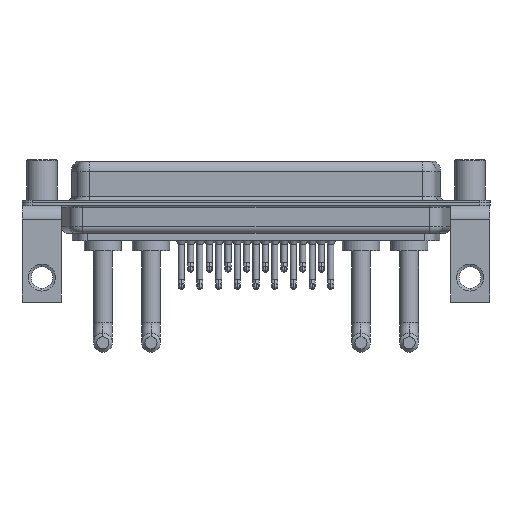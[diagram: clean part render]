
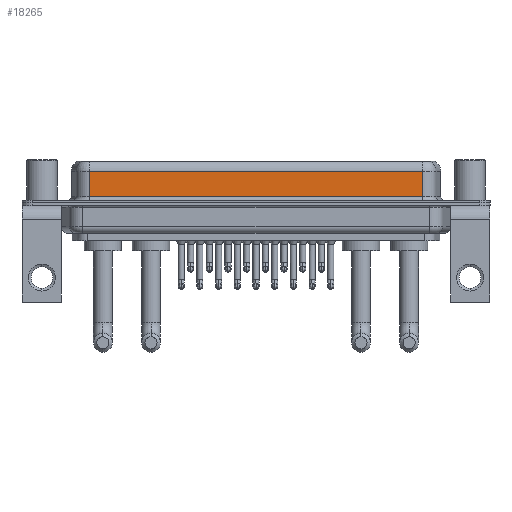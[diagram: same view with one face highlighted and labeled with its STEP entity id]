
A CAD part, front view. The second image highlights one B-rep face of the part: STEP entity #18265.
In plain terms, the highlighted planar face has unit normal (0, -1, 0).
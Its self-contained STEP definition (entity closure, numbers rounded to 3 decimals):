
#540 = VECTOR ( 'NONE', #15277, 1000. ) ;
#2119 = EDGE_LOOP ( 'NONE', ( #23455, #6418, #21085, #22426 ) ) ;
#3664 = AXIS2_PLACEMENT_3D ( 'NONE', #14513, #5076, #12653 ) ;
#4736 = DIRECTION ( 'NONE',  ( -1., 0., 0. ) ) ;
#5076 = DIRECTION ( 'NONE',  ( 0., 1., 0. ) ) ;
#5312 = CARTESIAN_POINT ( 'NONE',  ( 56.462, -3.95, 0.9 ) ) ;
#5611 = CARTESIAN_POINT ( 'NONE',  ( 56.462, -3.95, 6.4 ) ) ;
#6130 = LINE ( 'NONE', #19630, #22427 ) ;
#6417 = EDGE_CURVE ( 'NONE', #24205, #14981, #13853, .T. ) ;
#6418 = ORIENTED_EDGE ( 'NONE', *, *, #17570, .T. ) ;
#7288 = VERTEX_POINT ( 'NONE', #24466 ) ;
#8151 = CARTESIAN_POINT ( 'NONE',  ( 7.038, -3.95, 6.4 ) ) ;
#8830 = PLANE ( 'NONE',  #3664 ) ;
#9139 = CARTESIAN_POINT ( 'NONE',  ( 56.462, -3.95, 4.65 ) ) ;
#9355 = LINE ( 'NONE', #5611, #540 ) ;
#10412 = CARTESIAN_POINT ( 'NONE',  ( 7.038, -3.95, 0.9 ) ) ;
#10696 = FACE_OUTER_BOUND ( 'NONE', #2119, .T. ) ;
#11996 = DIRECTION ( 'NONE',  ( 1., 0., 0. ) ) ;
#12653 = DIRECTION ( 'NONE',  ( 0., 0., 1. ) ) ;
#13569 = EDGE_CURVE ( 'NONE', #17259, #14981, #9355, .T. ) ;
#13853 = LINE ( 'NONE', #23278, #16533 ) ;
#14073 = LINE ( 'NONE', #8151, #21169 ) ;
#14354 = EDGE_CURVE ( 'NONE', #7288, #24205, #14073, .T. ) ;
#14513 = CARTESIAN_POINT ( 'NONE',  ( 56.462, -3.95, 6.4 ) ) ;
#14981 = VERTEX_POINT ( 'NONE', #5312 ) ;
#15277 = DIRECTION ( 'NONE',  ( 0., 0., -1. ) ) ;
#16533 = VECTOR ( 'NONE', #11996, 1000. ) ;
#17259 = VERTEX_POINT ( 'NONE', #9139 ) ;
#17570 = EDGE_CURVE ( 'NONE', #17259, #7288, #6130, .T. ) ;
#18265 = ADVANCED_FACE ( 'NONE', ( #10696 ), #8830, .F. ) ;
#19630 = CARTESIAN_POINT ( 'NONE',  ( 56.462, -3.95, 4.65 ) ) ;
#21085 = ORIENTED_EDGE ( 'NONE', *, *, #14354, .T. ) ;
#21169 = VECTOR ( 'NONE', #21394, 1000. ) ;
#21394 = DIRECTION ( 'NONE',  ( 0., 0., -1. ) ) ;
#22426 = ORIENTED_EDGE ( 'NONE', *, *, #6417, .T. ) ;
#22427 = VECTOR ( 'NONE', #4736, 1000. ) ;
#23278 = CARTESIAN_POINT ( 'NONE',  ( 56.462, -3.95, 0.9 ) ) ;
#23455 = ORIENTED_EDGE ( 'NONE', *, *, #13569, .F. ) ;
#24205 = VERTEX_POINT ( 'NONE', #10412 ) ;
#24466 = CARTESIAN_POINT ( 'NONE',  ( 7.038, -3.95, 4.65 ) ) ;
